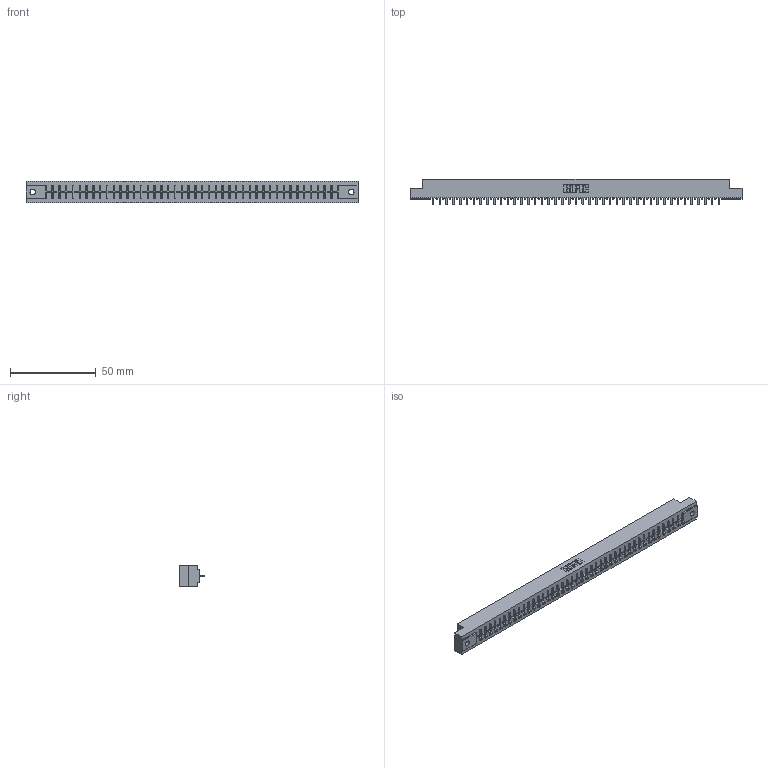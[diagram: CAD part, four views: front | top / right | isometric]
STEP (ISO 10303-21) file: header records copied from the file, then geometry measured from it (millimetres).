
FILE_DESCRIPTION (( 'STEP AP203' ), '1' );
FILE_NAME ('316-043-521-102.STEP', '2018-07-31T06:05:03', ( '' ), ( '' ), 'SwSTEP 2.0', 'SolidWorks 2016', '' );
FILE_SCHEMA (( 'CONFIG_CONTROL_DESIGN' ));
Length unit declared in the file: inch
Products named in the file (3): 316-043-521-102; 306 Part_.128 Dia; 306-290-001_121
Assembly tree (44 placements, depth 2):
  316-043-521-102
    306 Part_.128 Dia
    306-290-001_121  x43
Bounding box: 193.4 x 14.88 x 12.7 mm (x, y, z)
Volume: 21313.1 mm3; surface area: 21284.1 mm2
Topology: 44 solids, 44 shells, 3126 faces, 8787 edges, 5626 vertices
Faces by surface type: plane 2089, cylinder 865, sphere 172
Entity records: 39928 total; most frequent: CARTESIAN_POINT 6704, ORIENTED_EDGE 6646, DIRECTION 6611, EDGE_CURVE 3323, LINE 2601, VECTOR 2601, VERTEX_POINT 2098, AXIS2_PLACEMENT_3D 2005
